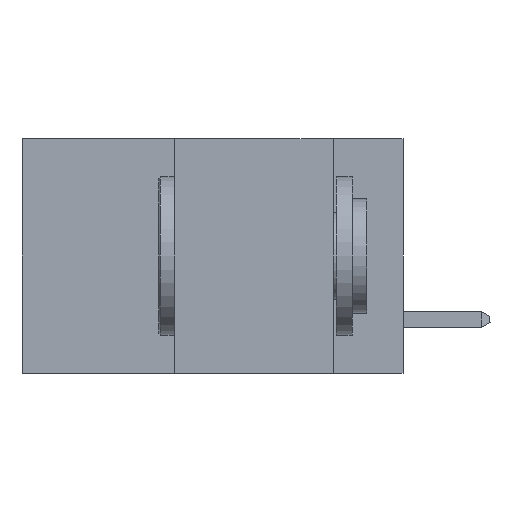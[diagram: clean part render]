
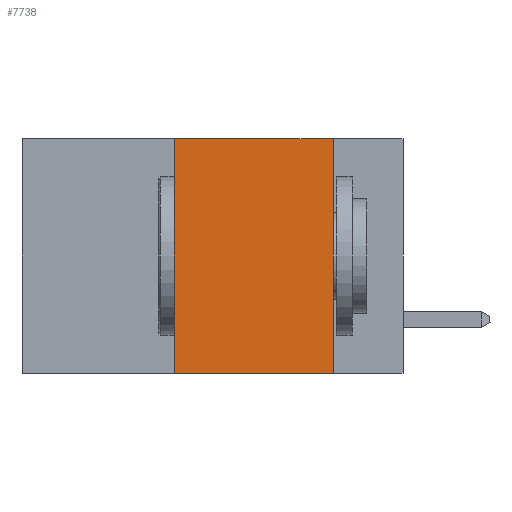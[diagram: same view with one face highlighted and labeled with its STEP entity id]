
A CAD part, left-side view. The second image highlights one B-rep face of the part: STEP entity #7738.
In plain terms, the highlighted planar face has unit normal (-1, 0, 0).
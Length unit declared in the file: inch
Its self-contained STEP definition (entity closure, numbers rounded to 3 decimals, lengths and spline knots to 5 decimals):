
#1161 = CARTESIAN_POINT ( 'NONE',  ( 0., 0.11, 0. ) ) ;
#1238 = LINE ( 'NONE', #18525, #17725 ) ;
#1301 = DIRECTION ( 'NONE',  ( 0., 0., 1. ) ) ;
#1387 = DIRECTION ( 'NONE',  ( 0., 0., -1. ) ) ;
#2893 = ORIENTED_EDGE ( 'NONE', *, *, #13012, .T. ) ;
#2899 = LINE ( 'NONE', #3361, #19342 ) ;
#2998 = FACE_OUTER_BOUND ( 'NONE', #16584, .T. ) ;
#3361 = CARTESIAN_POINT ( 'NONE',  ( 0., 0.6, 0. ) ) ;
#4525 = CARTESIAN_POINT ( 'NONE',  ( 0., 0.6, 0. ) ) ;
#6168 = CARTESIAN_POINT ( 'NONE',  ( 0., 0.36, -0.37 ) ) ;
#6258 = CARTESIAN_POINT ( 'NONE',  ( 0., 0.11, 0. ) ) ;
#7465 = DIRECTION ( 'NONE',  ( 0., -1., 0. ) ) ;
#7738 = ADVANCED_FACE ( 'NONE', ( #2998 ), #7856, .F. ) ;
#7856 = PLANE ( 'NONE',  #15015 ) ;
#7910 = VERTEX_POINT ( 'NONE', #17652 ) ;
#8112 = DIRECTION ( 'NONE',  ( 0., -1., 0. ) ) ;
#8594 = LINE ( 'NONE', #12491, #14317 ) ;
#9373 = LINE ( 'NONE', #6258, #11340 ) ;
#10382 = CARTESIAN_POINT ( 'NONE',  ( 0., 0.11, -0.37 ) ) ;
#10512 = EDGE_CURVE ( 'NONE', #16533, #19313, #9373, .T. ) ;
#11340 = VECTOR ( 'NONE', #15725, 39.37008 ) ;
#12491 = CARTESIAN_POINT ( 'NONE',  ( 0., 0.36, 0. ) ) ;
#13012 = EDGE_CURVE ( 'NONE', #20378, #19313, #1238, .T. ) ;
#14086 = ORIENTED_EDGE ( 'NONE', *, *, #17412, .F. ) ;
#14317 = VECTOR ( 'NONE', #1301, 39.37008 ) ;
#15015 = AXIS2_PLACEMENT_3D ( 'NONE', #4525, #15856, #1387 ) ;
#15725 = DIRECTION ( 'NONE',  ( 0., 0., -1. ) ) ;
#15856 = DIRECTION ( 'NONE',  ( 1., 0., 0. ) ) ;
#16386 = ORIENTED_EDGE ( 'NONE', *, *, #10512, .F. ) ;
#16533 = VERTEX_POINT ( 'NONE', #1161 ) ;
#16584 = EDGE_LOOP ( 'NONE', ( #16386, #14086, #18820, #2893 ) ) ;
#17412 = EDGE_CURVE ( 'NONE', #7910, #16533, #2899, .T. ) ;
#17652 = CARTESIAN_POINT ( 'NONE',  ( 0., 0.36, 0. ) ) ;
#17725 = VECTOR ( 'NONE', #7465, 39.37008 ) ;
#18525 = CARTESIAN_POINT ( 'NONE',  ( 0., 0.6, -0.37 ) ) ;
#18820 = ORIENTED_EDGE ( 'NONE', *, *, #19977, .F. ) ;
#19313 = VERTEX_POINT ( 'NONE', #10382 ) ;
#19342 = VECTOR ( 'NONE', #8112, 39.37008 ) ;
#19977 = EDGE_CURVE ( 'NONE', #20378, #7910, #8594, .T. ) ;
#20378 = VERTEX_POINT ( 'NONE', #6168 ) ;
